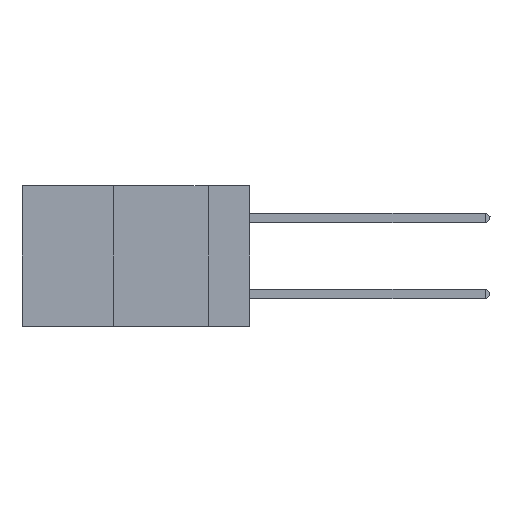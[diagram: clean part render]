
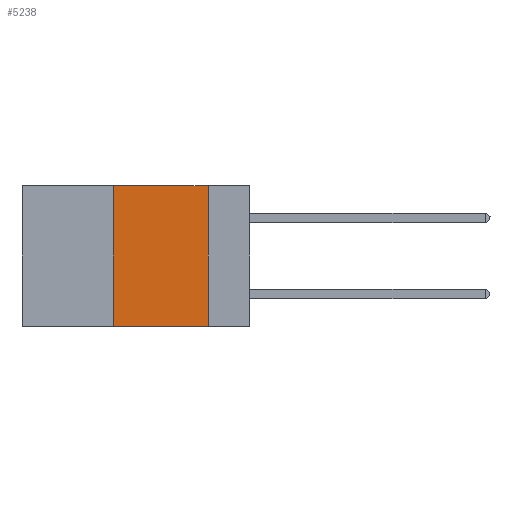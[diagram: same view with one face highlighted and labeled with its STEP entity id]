
A CAD part, left-side view. The second image highlights one B-rep face of the part: STEP entity #5238.
In plain terms, the highlighted planar face has unit normal (-1, 0, 0).
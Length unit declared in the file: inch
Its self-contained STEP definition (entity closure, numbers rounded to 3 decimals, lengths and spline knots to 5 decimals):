
#1201 = CARTESIAN_POINT ( 'NONE',  ( 0., 0.36, 0. ) ) ;
#1405 = CARTESIAN_POINT ( 'NONE',  ( 0., 0.6, 0. ) ) ;
#1642 = ORIENTED_EDGE ( 'NONE', *, *, #7268, .F. ) ;
#2066 = AXIS2_PLACEMENT_3D ( 'NONE', #1405, #23627, #10787 ) ;
#2143 = EDGE_CURVE ( 'NONE', #11054, #18535, #16865, .T. ) ;
#2264 = ORIENTED_EDGE ( 'NONE', *, *, #8538, .F. ) ;
#3295 = PLANE ( 'NONE',  #2066 ) ;
#4154 = CARTESIAN_POINT ( 'NONE',  ( 0., 0.36, -0.37 ) ) ;
#5238 = ADVANCED_FACE ( 'NONE', ( #19393 ), #3295, .F. ) ;
#5596 = ORIENTED_EDGE ( 'NONE', *, *, #2143, .T. ) ;
#6593 = DIRECTION ( 'NONE',  ( 0., -1., 0. ) ) ;
#7268 = EDGE_CURVE ( 'NONE', #22978, #18535, #12113, .T. ) ;
#8256 = VECTOR ( 'NONE', #6593, 39.37008 ) ;
#8538 = EDGE_CURVE ( 'NONE', #11054, #15024, #12041, .T. ) ;
#8806 = CARTESIAN_POINT ( 'NONE',  ( 0., 0.36, 0. ) ) ;
#9257 = CARTESIAN_POINT ( 'NONE',  ( 0., 0.6, -0.37 ) ) ;
#10787 = DIRECTION ( 'NONE',  ( 0., 0., -1. ) ) ;
#11054 = VERTEX_POINT ( 'NONE', #4154 ) ;
#11757 = ORIENTED_EDGE ( 'NONE', *, *, #14614, .F. ) ;
#12041 = LINE ( 'NONE', #8806, #22475 ) ;
#12113 = LINE ( 'NONE', #17434, #23687 ) ;
#12755 = DIRECTION ( 'NONE',  ( 0., -1., 0. ) ) ;
#14530 = CARTESIAN_POINT ( 'NONE',  ( 0., 0.11, 0. ) ) ;
#14537 = VECTOR ( 'NONE', #12755, 39.37008 ) ;
#14614 = EDGE_CURVE ( 'NONE', #15024, #22978, #14643, .T. ) ;
#14643 = LINE ( 'NONE', #15686, #8256 ) ;
#15024 = VERTEX_POINT ( 'NONE', #1201 ) ;
#15686 = CARTESIAN_POINT ( 'NONE',  ( 0., 0.6, 0. ) ) ;
#16262 = CARTESIAN_POINT ( 'NONE',  ( 0., 0.11, -0.37 ) ) ;
#16844 = DIRECTION ( 'NONE',  ( 0., 0., 1. ) ) ;
#16865 = LINE ( 'NONE', #9257, #14537 ) ;
#17434 = CARTESIAN_POINT ( 'NONE',  ( 0., 0.11, 0. ) ) ;
#18535 = VERTEX_POINT ( 'NONE', #16262 ) ;
#19258 = EDGE_LOOP ( 'NONE', ( #1642, #11757, #2264, #5596 ) ) ;
#19393 = FACE_OUTER_BOUND ( 'NONE', #19258, .T. ) ;
#20844 = DIRECTION ( 'NONE',  ( 0., 0., -1. ) ) ;
#22475 = VECTOR ( 'NONE', #16844, 39.37008 ) ;
#22978 = VERTEX_POINT ( 'NONE', #14530 ) ;
#23627 = DIRECTION ( 'NONE',  ( 1., 0., 0. ) ) ;
#23687 = VECTOR ( 'NONE', #20844, 39.37008 ) ;
